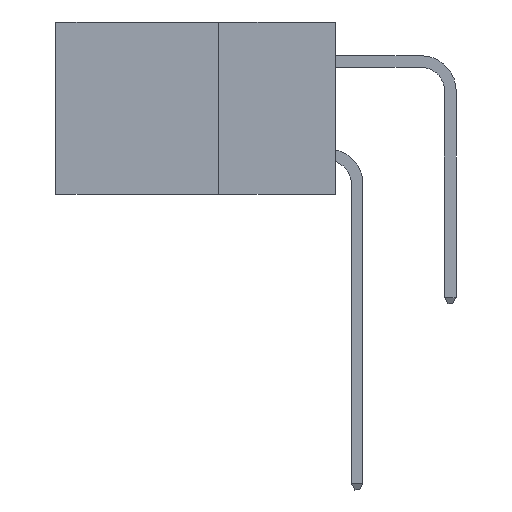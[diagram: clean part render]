
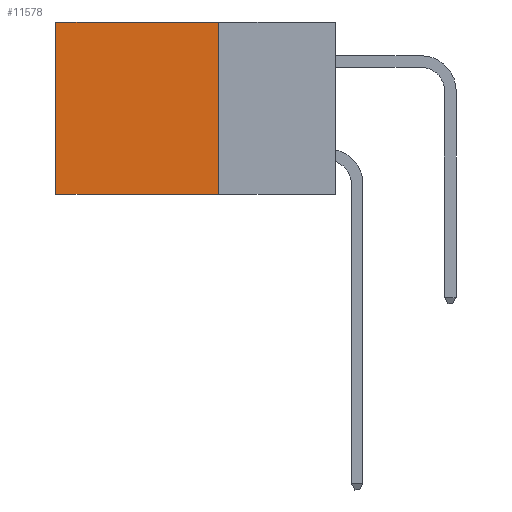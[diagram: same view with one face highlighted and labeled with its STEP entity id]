
A CAD part, left-side view. The second image highlights one B-rep face of the part: STEP entity #11578.
In plain terms, the highlighted planar face has unit normal (-1, 0, 0).
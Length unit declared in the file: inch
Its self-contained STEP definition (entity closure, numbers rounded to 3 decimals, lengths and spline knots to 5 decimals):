
#100 = PLANE ( 'NONE',  #13286 ) ;
#453 = CARTESIAN_POINT ( 'NONE',  ( 0.2875, 0.25, 0. ) ) ;
#464 = LINE ( 'NONE', #14300, #5988 ) ;
#563 = ORIENTED_EDGE ( 'NONE', *, *, #2770, .T. ) ;
#604 = VERTEX_POINT ( 'NONE', #453 ) ;
#867 = VERTEX_POINT ( 'NONE', #10572 ) ;
#1356 = ORIENTED_EDGE ( 'NONE', *, *, #14553, .F. ) ;
#1429 = ORIENTED_EDGE ( 'NONE', *, *, #8678, .T. ) ;
#1725 = DIRECTION ( 'NONE',  ( 0., 0., -1. ) ) ;
#2182 = LINE ( 'NONE', #2612, #2921 ) ;
#2612 = CARTESIAN_POINT ( 'NONE',  ( 0.2875, 0.25, -0.37 ) ) ;
#2770 = EDGE_CURVE ( 'NONE', #604, #5311, #464, .T. ) ;
#2921 = VECTOR ( 'NONE', #9796, 39.37008 ) ;
#4262 = CARTESIAN_POINT ( 'NONE',  ( 0.2875, 0.6, 0. ) ) ;
#5037 = VECTOR ( 'NONE', #1725, 39.37008 ) ;
#5311 = VERTEX_POINT ( 'NONE', #5816 ) ;
#5816 = CARTESIAN_POINT ( 'NONE',  ( 0.2875, 0.6, 0. ) ) ;
#5988 = VECTOR ( 'NONE', #7155, 39.37008 ) ;
#6329 = EDGE_CURVE ( 'NONE', #604, #867, #8575, .T. ) ;
#7155 = DIRECTION ( 'NONE',  ( 0., 1., 0. ) ) ;
#8559 = DIRECTION ( 'NONE',  ( 0., 0., -1. ) ) ;
#8575 = LINE ( 'NONE', #14515, #11941 ) ;
#8622 = CARTESIAN_POINT ( 'NONE',  ( 0.2875, 0.25, 0. ) ) ;
#8678 = EDGE_CURVE ( 'NONE', #5311, #11761, #9992, .T. ) ;
#9796 = DIRECTION ( 'NONE',  ( 0., 1., 0. ) ) ;
#9992 = LINE ( 'NONE', #4262, #5037 ) ;
#10191 = ORIENTED_EDGE ( 'NONE', *, *, #6329, .F. ) ;
#10572 = CARTESIAN_POINT ( 'NONE',  ( 0.2875, 0.25, -0.37 ) ) ;
#11118 = DIRECTION ( 'NONE',  ( 0., 0., -1. ) ) ;
#11578 = ADVANCED_FACE ( 'NONE', ( #13659 ), #100, .F. ) ;
#11761 = VERTEX_POINT ( 'NONE', #12749 ) ;
#11941 = VECTOR ( 'NONE', #8559, 39.37008 ) ;
#12749 = CARTESIAN_POINT ( 'NONE',  ( 0.2875, 0.6, -0.37 ) ) ;
#13286 = AXIS2_PLACEMENT_3D ( 'NONE', #8622, #13443, #11118 ) ;
#13443 = DIRECTION ( 'NONE',  ( 1., 0., 0. ) ) ;
#13659 = FACE_OUTER_BOUND ( 'NONE', #14260, .T. ) ;
#14260 = EDGE_LOOP ( 'NONE', ( #1429, #1356, #10191, #563 ) ) ;
#14300 = CARTESIAN_POINT ( 'NONE',  ( 0.2875, 0.25, 0. ) ) ;
#14515 = CARTESIAN_POINT ( 'NONE',  ( 0.2875, 0.25, 0. ) ) ;
#14553 = EDGE_CURVE ( 'NONE', #867, #11761, #2182, .T. ) ;
